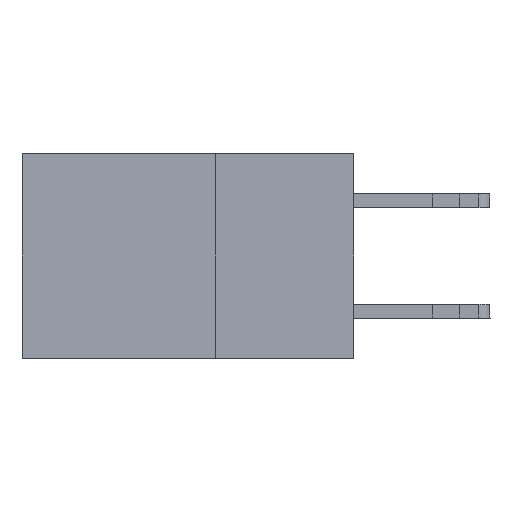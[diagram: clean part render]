
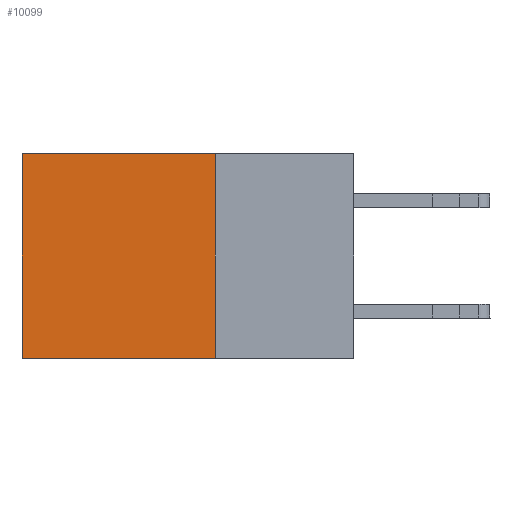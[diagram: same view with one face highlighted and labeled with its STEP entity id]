
A CAD part, left-side view. The second image highlights one B-rep face of the part: STEP entity #10099.
In plain terms, the highlighted planar face has unit normal (-1, 0, 0).
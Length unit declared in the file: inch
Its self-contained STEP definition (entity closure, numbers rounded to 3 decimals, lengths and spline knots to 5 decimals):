
#944 = LINE ( 'NONE', #12451, #15309 ) ;
#1188 = LINE ( 'NONE', #5022, #11741 ) ;
#2089 = VERTEX_POINT ( 'NONE', #16259 ) ;
#2147 = EDGE_CURVE ( 'NONE', #16741, #16648, #944, .T. ) ;
#2267 = DIRECTION ( 'NONE',  ( 1., 0., 0. ) ) ;
#2650 = VECTOR ( 'NONE', #14414, 39.37008 ) ;
#3132 = CARTESIAN_POINT ( 'NONE',  ( 0.2875, 0.25, 0. ) ) ;
#5022 = CARTESIAN_POINT ( 'NONE',  ( 0.2875, 0.25, 0. ) ) ;
#5232 = FACE_OUTER_BOUND ( 'NONE', #14655, .T. ) ;
#6570 = EDGE_CURVE ( 'NONE', #8902, #2089, #1188, .T. ) ;
#7043 = DIRECTION ( 'NONE',  ( 0., 0., -1. ) ) ;
#7703 = PLANE ( 'NONE',  #13528 ) ;
#7806 = CARTESIAN_POINT ( 'NONE',  ( 0.2875, 0.6, -0.37 ) ) ;
#8731 = ORIENTED_EDGE ( 'NONE', *, *, #16445, .F. ) ;
#8783 = ORIENTED_EDGE ( 'NONE', *, *, #9272, .T. ) ;
#8902 = VERTEX_POINT ( 'NONE', #3132 ) ;
#9272 = EDGE_CURVE ( 'NONE', #8902, #16741, #13727, .T. ) ;
#10099 = ADVANCED_FACE ( 'NONE', ( #5232 ), #7703, .F. ) ;
#10437 = CARTESIAN_POINT ( 'NONE',  ( 0.2875, 0.25, 0. ) ) ;
#11591 = DIRECTION ( 'NONE',  ( 0., 1., 0. ) ) ;
#11741 = VECTOR ( 'NONE', #13302, 39.37008 ) ;
#11862 = DIRECTION ( 'NONE',  ( 0., 0., -1. ) ) ;
#12158 = LINE ( 'NONE', #12953, #15502 ) ;
#12166 = CARTESIAN_POINT ( 'NONE',  ( 0.2875, 0.6, 0. ) ) ;
#12451 = CARTESIAN_POINT ( 'NONE',  ( 0.2875, 0.6, 0. ) ) ;
#12477 = ORIENTED_EDGE ( 'NONE', *, *, #6570, .F. ) ;
#12695 = ORIENTED_EDGE ( 'NONE', *, *, #2147, .T. ) ;
#12953 = CARTESIAN_POINT ( 'NONE',  ( 0.2875, 0.25, -0.37 ) ) ;
#13302 = DIRECTION ( 'NONE',  ( 0., 0., -1. ) ) ;
#13528 = AXIS2_PLACEMENT_3D ( 'NONE', #10437, #2267, #11862 ) ;
#13727 = LINE ( 'NONE', #14351, #2650 ) ;
#14351 = CARTESIAN_POINT ( 'NONE',  ( 0.2875, 0.25, 0. ) ) ;
#14414 = DIRECTION ( 'NONE',  ( 0., 1., 0. ) ) ;
#14655 = EDGE_LOOP ( 'NONE', ( #12695, #8731, #12477, #8783 ) ) ;
#15309 = VECTOR ( 'NONE', #7043, 39.37008 ) ;
#15502 = VECTOR ( 'NONE', #11591, 39.37008 ) ;
#16259 = CARTESIAN_POINT ( 'NONE',  ( 0.2875, 0.25, -0.37 ) ) ;
#16445 = EDGE_CURVE ( 'NONE', #2089, #16648, #12158, .T. ) ;
#16648 = VERTEX_POINT ( 'NONE', #7806 ) ;
#16741 = VERTEX_POINT ( 'NONE', #12166 ) ;
